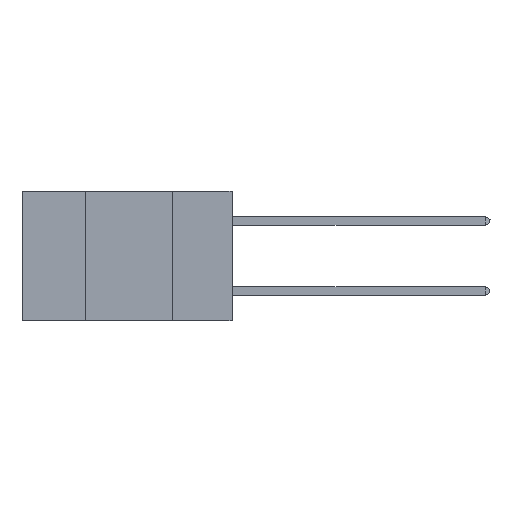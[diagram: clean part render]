
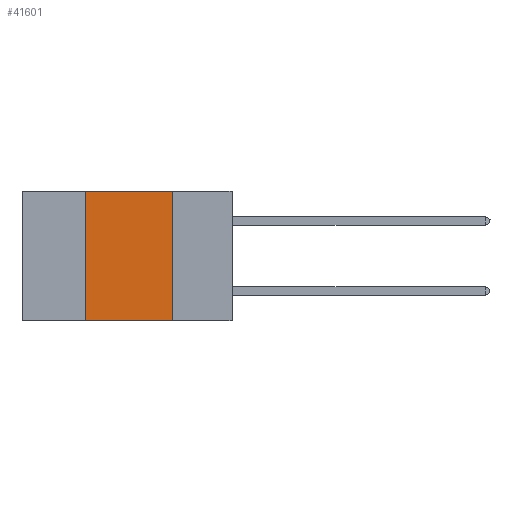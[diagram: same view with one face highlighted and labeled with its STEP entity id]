
A CAD part, left-side view. The second image highlights one B-rep face of the part: STEP entity #41601.
In plain terms, the highlighted planar face has unit normal (-1, 0, 0).
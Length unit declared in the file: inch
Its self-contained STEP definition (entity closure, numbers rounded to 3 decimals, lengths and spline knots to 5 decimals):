
#161 = VERTEX_POINT ( 'NONE', #32696 ) ;
#1443 = VERTEX_POINT ( 'NONE', #27316 ) ;
#2144 = LINE ( 'NONE', #15443, #11050 ) ;
#2670 = ORIENTED_EDGE ( 'NONE', *, *, #15938, .T. ) ;
#2749 = LINE ( 'NONE', #16060, #34605 ) ;
#2880 = ORIENTED_EDGE ( 'NONE', *, *, #4712, .F. ) ;
#4712 = EDGE_CURVE ( 'NONE', #18380, #161, #2749, .T. ) ;
#6664 = VERTEX_POINT ( 'NONE', #19939 ) ;
#6811 = LINE ( 'NONE', #36075, #36722 ) ;
#7795 = EDGE_LOOP ( 'NONE', ( #15393, #34684, #2880, #2670 ) ) ;
#8333 = VECTOR ( 'NONE', #17767, 39.37008 ) ;
#11050 = VECTOR ( 'NONE', #19592, 39.37008 ) ;
#11815 = PLANE ( 'NONE',  #36860 ) ;
#13689 = EDGE_CURVE ( 'NONE', #161, #6664, #6811, .T. ) ;
#14274 = LINE ( 'NONE', #28031, #8333 ) ;
#15393 = ORIENTED_EDGE ( 'NONE', *, *, #42893, .F. ) ;
#15443 = CARTESIAN_POINT ( 'NONE',  ( 0., 0.6, -0.37 ) ) ;
#15938 = EDGE_CURVE ( 'NONE', #18380, #1443, #2144, .T. ) ;
#16060 = CARTESIAN_POINT ( 'NONE',  ( 0., 0.42, 0. ) ) ;
#16916 = DIRECTION ( 'NONE',  ( 0., 0., 1. ) ) ;
#17081 = CARTESIAN_POINT ( 'NONE',  ( 0., 0.42, -0.37 ) ) ;
#17767 = DIRECTION ( 'NONE',  ( 0., 0., -1. ) ) ;
#17946 = DIRECTION ( 'NONE',  ( 0., 0., -1. ) ) ;
#18344 = DIRECTION ( 'NONE',  ( 1., 0., 0. ) ) ;
#18380 = VERTEX_POINT ( 'NONE', #17081 ) ;
#18571 = CARTESIAN_POINT ( 'NONE',  ( 0., 0.6, 0. ) ) ;
#19592 = DIRECTION ( 'NONE',  ( 0., -1., 0. ) ) ;
#19939 = CARTESIAN_POINT ( 'NONE',  ( 0., 0.17, 0. ) ) ;
#20138 = DIRECTION ( 'NONE',  ( 0., -1., 0. ) ) ;
#27316 = CARTESIAN_POINT ( 'NONE',  ( 0., 0.17, -0.37 ) ) ;
#28031 = CARTESIAN_POINT ( 'NONE',  ( 0., 0.17, 0. ) ) ;
#32696 = CARTESIAN_POINT ( 'NONE',  ( 0., 0.42, 0. ) ) ;
#34605 = VECTOR ( 'NONE', #16916, 39.37008 ) ;
#34684 = ORIENTED_EDGE ( 'NONE', *, *, #13689, .F. ) ;
#34752 = FACE_OUTER_BOUND ( 'NONE', #7795, .T. ) ;
#36075 = CARTESIAN_POINT ( 'NONE',  ( 0., 0.6, 0. ) ) ;
#36722 = VECTOR ( 'NONE', #20138, 39.37008 ) ;
#36860 = AXIS2_PLACEMENT_3D ( 'NONE', #18571, #18344, #17946 ) ;
#41601 = ADVANCED_FACE ( 'NONE', ( #34752 ), #11815, .F. ) ;
#42893 = EDGE_CURVE ( 'NONE', #6664, #1443, #14274, .T. ) ;
